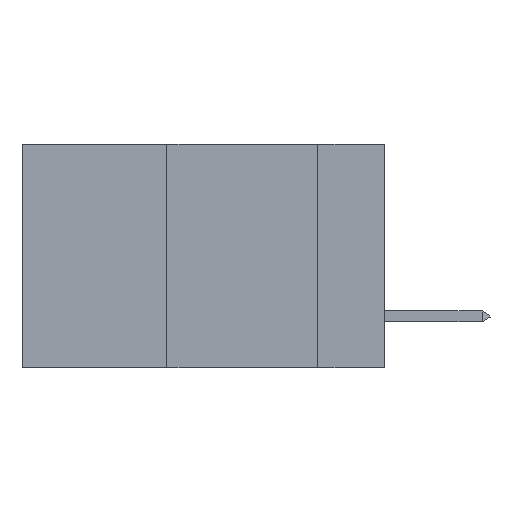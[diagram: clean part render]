
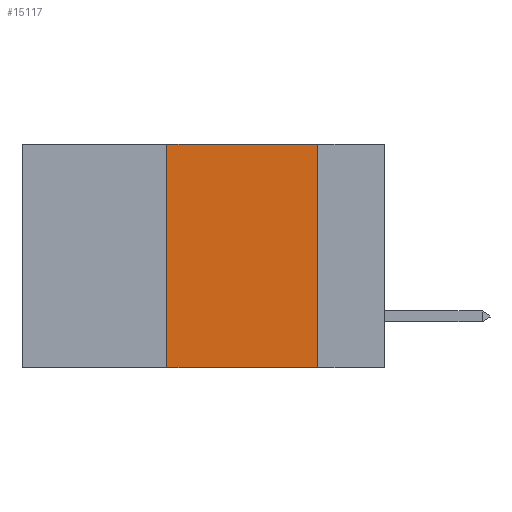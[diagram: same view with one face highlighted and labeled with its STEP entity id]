
A CAD part, left-side view. The second image highlights one B-rep face of the part: STEP entity #15117.
In plain terms, the highlighted planar face has unit normal (-1, 0, 0).
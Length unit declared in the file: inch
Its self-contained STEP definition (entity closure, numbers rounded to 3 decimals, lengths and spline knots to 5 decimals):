
#228 = VERTEX_POINT ( 'NONE', #3231 ) ;
#1601 = DIRECTION ( 'NONE',  ( 0., -1., 0. ) ) ;
#1652 = CARTESIAN_POINT ( 'NONE',  ( 0., 0.6, -0.37 ) ) ;
#1945 = FACE_OUTER_BOUND ( 'NONE', #5058, .T. ) ;
#1986 = PLANE ( 'NONE',  #6960 ) ;
#2042 = DIRECTION ( 'NONE',  ( 1., 0., 0. ) ) ;
#2606 = CARTESIAN_POINT ( 'NONE',  ( 0., 0.11, 0. ) ) ;
#2877 = VERTEX_POINT ( 'NONE', #8445 ) ;
#3231 = CARTESIAN_POINT ( 'NONE',  ( 0., 0.11, 0. ) ) ;
#3914 = VECTOR ( 'NONE', #1601, 39.37008 ) ;
#3930 = DIRECTION ( 'NONE',  ( 0., 0., 1. ) ) ;
#4349 = EDGE_CURVE ( 'NONE', #16734, #228, #8471, .T. ) ;
#4839 = VECTOR ( 'NONE', #6193, 39.37008 ) ;
#4985 = EDGE_CURVE ( 'NONE', #8428, #16734, #10985, .T. ) ;
#4987 = CARTESIAN_POINT ( 'NONE',  ( 0., 0.6, 0. ) ) ;
#5058 = EDGE_LOOP ( 'NONE', ( #15203, #8232, #17275, #16643 ) ) ;
#6193 = DIRECTION ( 'NONE',  ( 0., -1., 0. ) ) ;
#6320 = VECTOR ( 'NONE', #3930, 39.37008 ) ;
#6960 = AXIS2_PLACEMENT_3D ( 'NONE', #11603, #2042, #11788 ) ;
#8232 = ORIENTED_EDGE ( 'NONE', *, *, #4349, .F. ) ;
#8428 = VERTEX_POINT ( 'NONE', #13828 ) ;
#8445 = CARTESIAN_POINT ( 'NONE',  ( 0., 0.11, -0.37 ) ) ;
#8471 = LINE ( 'NONE', #4987, #4839 ) ;
#9380 = EDGE_CURVE ( 'NONE', #228, #2877, #15479, .T. ) ;
#9889 = CARTESIAN_POINT ( 'NONE',  ( 0., 0.36, 0. ) ) ;
#10696 = EDGE_CURVE ( 'NONE', #8428, #2877, #15217, .T. ) ;
#10985 = LINE ( 'NONE', #13433, #6320 ) ;
#11027 = VECTOR ( 'NONE', #12294, 39.37008 ) ;
#11603 = CARTESIAN_POINT ( 'NONE',  ( 0., 0.6, 0. ) ) ;
#11788 = DIRECTION ( 'NONE',  ( 0., 0., -1. ) ) ;
#12294 = DIRECTION ( 'NONE',  ( 0., 0., -1. ) ) ;
#13433 = CARTESIAN_POINT ( 'NONE',  ( 0., 0.36, 0. ) ) ;
#13828 = CARTESIAN_POINT ( 'NONE',  ( 0., 0.36, -0.37 ) ) ;
#15117 = ADVANCED_FACE ( 'NONE', ( #1945 ), #1986, .F. ) ;
#15203 = ORIENTED_EDGE ( 'NONE', *, *, #9380, .F. ) ;
#15217 = LINE ( 'NONE', #1652, #3914 ) ;
#15479 = LINE ( 'NONE', #2606, #11027 ) ;
#16643 = ORIENTED_EDGE ( 'NONE', *, *, #10696, .T. ) ;
#16734 = VERTEX_POINT ( 'NONE', #9889 ) ;
#17275 = ORIENTED_EDGE ( 'NONE', *, *, #4985, .F. ) ;
